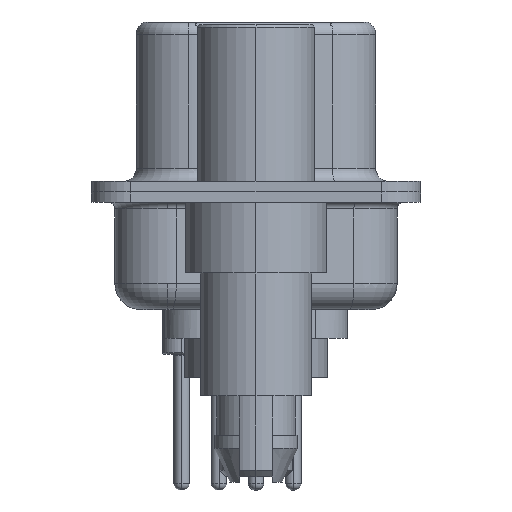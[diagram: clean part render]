
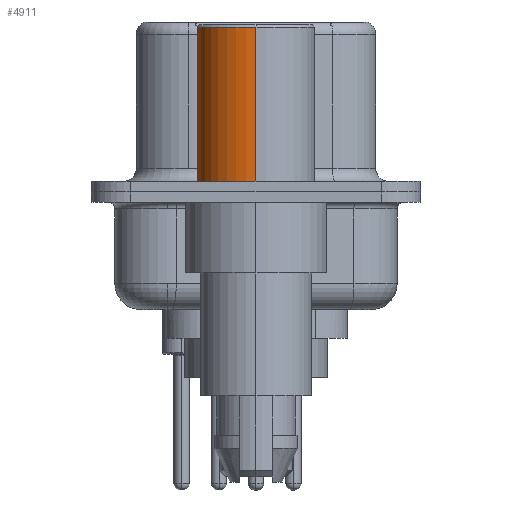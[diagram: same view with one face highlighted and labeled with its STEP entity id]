
A CAD part, left-side view. The second image highlights one B-rep face of the part: STEP entity #4911.
In plain terms, the highlighted cylindrical face has radius 2.25 mm (diameter 4.5 mm), a partial arc.
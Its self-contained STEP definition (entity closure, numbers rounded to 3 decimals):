
#710 = DIRECTION ( 'NONE',  ( 1., 0., 0. ) ) ;
#2089 = LINE ( 'NONE', #14231, #22907 ) ;
#2629 = EDGE_CURVE ( 'NONE', #4666, #16846, #18961, .T. ) ;
#2785 = ORIENTED_EDGE ( 'NONE', *, *, #12062, .T. ) ;
#4369 = VECTOR ( 'NONE', #6718, 1000. ) ;
#4666 = VERTEX_POINT ( 'NONE', #16475 ) ;
#4732 = EDGE_LOOP ( 'NONE', ( #2785, #16651, #7348, #22088 ) ) ;
#4911 = ADVANCED_FACE ( 'NONE', ( #9038 ), #19077, .T. ) ;
#6202 = DIRECTION ( 'NONE',  ( 1., 0., 0. ) ) ;
#6718 = DIRECTION ( 'NONE',  ( 0., 0., 1. ) ) ;
#6724 = AXIS2_PLACEMENT_3D ( 'NONE', #21384, #21726, #710 ) ;
#6955 = CARTESIAN_POINT ( 'NONE',  ( -2.25, 0., 6.3 ) ) ;
#7348 = ORIENTED_EDGE ( 'NONE', *, *, #2629, .F. ) ;
#7656 = CARTESIAN_POINT ( 'NONE',  ( -2.25, 0., 0.4 ) ) ;
#8062 = VERTEX_POINT ( 'NONE', #7656 ) ;
#9038 = FACE_OUTER_BOUND ( 'NONE', #4732, .T. ) ;
#11370 = CARTESIAN_POINT ( 'NONE',  ( 2.25, 0., 0.4 ) ) ;
#11665 = DIRECTION ( 'NONE',  ( 0., 0., 1. ) ) ;
#12062 = EDGE_CURVE ( 'NONE', #22617, #8062, #18384, .T. ) ;
#14231 = CARTESIAN_POINT ( 'NONE',  ( 2.25, 0., 0.581 ) ) ;
#14436 = LINE ( 'NONE', #20798, #4369 ) ;
#14856 = AXIS2_PLACEMENT_3D ( 'NONE', #19410, #20799, #6202 ) ;
#16135 = EDGE_CURVE ( 'NONE', #8062, #16846, #14436, .T. ) ;
#16475 = CARTESIAN_POINT ( 'NONE',  ( 2.25, 0., 6.3 ) ) ;
#16651 = ORIENTED_EDGE ( 'NONE', *, *, #16135, .T. ) ;
#16846 = VERTEX_POINT ( 'NONE', #6955 ) ;
#16964 = EDGE_CURVE ( 'NONE', #22617, #4666, #2089, .T. ) ;
#18384 = CIRCLE ( 'NONE', #20074, 2.25 ) ;
#18961 = CIRCLE ( 'NONE', #6724, 2.25 ) ;
#19077 = CYLINDRICAL_SURFACE ( 'NONE', #14856, 2.25 ) ;
#19410 = CARTESIAN_POINT ( 'NONE',  ( 0., 0., 0.581 ) ) ;
#20074 = AXIS2_PLACEMENT_3D ( 'NONE', #23751, #11665, #25772 ) ;
#20306 = DIRECTION ( 'NONE',  ( 0., 0., 1. ) ) ;
#20798 = CARTESIAN_POINT ( 'NONE',  ( -2.25, 0., 0.581 ) ) ;
#20799 = DIRECTION ( 'NONE',  ( 0., 0., 1. ) ) ;
#21384 = CARTESIAN_POINT ( 'NONE',  ( 0., 0., 6.3 ) ) ;
#21726 = DIRECTION ( 'NONE',  ( 0., 0., 1. ) ) ;
#22088 = ORIENTED_EDGE ( 'NONE', *, *, #16964, .F. ) ;
#22617 = VERTEX_POINT ( 'NONE', #11370 ) ;
#22907 = VECTOR ( 'NONE', #20306, 1000. ) ;
#23751 = CARTESIAN_POINT ( 'NONE',  ( 0., 0., 0.4 ) ) ;
#25772 = DIRECTION ( 'NONE',  ( 1., 0., 0. ) ) ;
